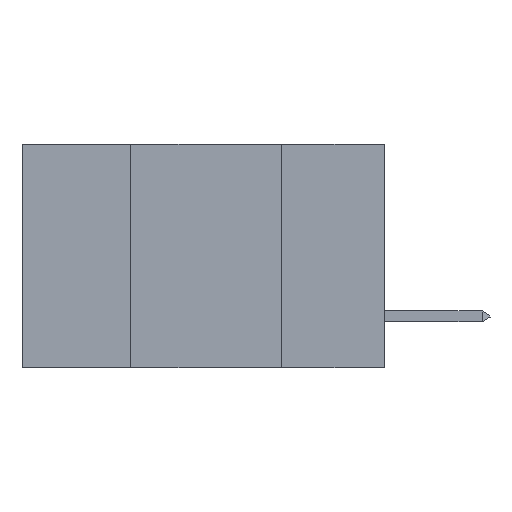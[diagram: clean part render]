
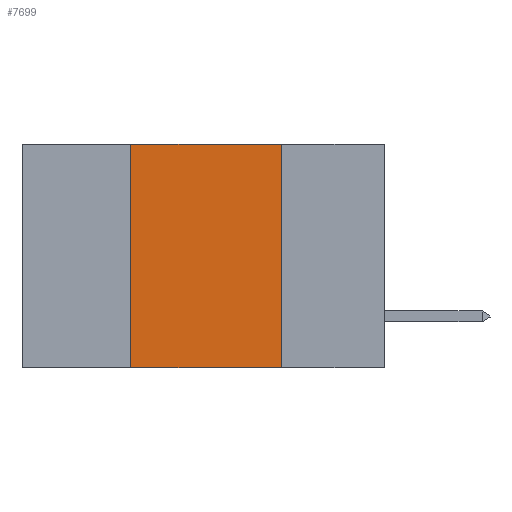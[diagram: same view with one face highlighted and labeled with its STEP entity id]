
A CAD part, left-side view. The second image highlights one B-rep face of the part: STEP entity #7699.
In plain terms, the highlighted planar face has unit normal (-1, 0, 0).
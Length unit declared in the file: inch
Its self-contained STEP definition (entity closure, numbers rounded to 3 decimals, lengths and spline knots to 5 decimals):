
#164 = DIRECTION ( 'NONE',  ( 0., -1., 0. ) ) ;
#197 = LINE ( 'NONE', #2071, #16252 ) ;
#1173 = ORIENTED_EDGE ( 'NONE', *, *, #15285, .T. ) ;
#2071 = CARTESIAN_POINT ( 'NONE',  ( 0., 0.42, 0. ) ) ;
#2928 = EDGE_CURVE ( 'NONE', #18189, #19625, #12717, .T. ) ;
#3046 = DIRECTION ( 'NONE',  ( 0., -1., 0. ) ) ;
#3427 = ORIENTED_EDGE ( 'NONE', *, *, #17826, .F. ) ;
#3479 = VECTOR ( 'NONE', #3046, 39.37008 ) ;
#3629 = DIRECTION ( 'NONE',  ( 0., 0., 1. ) ) ;
#4504 = VERTEX_POINT ( 'NONE', #11146 ) ;
#5910 = CARTESIAN_POINT ( 'NONE',  ( 0., 0.17, 0. ) ) ;
#6726 = ORIENTED_EDGE ( 'NONE', *, *, #8571, .F. ) ;
#6956 = LINE ( 'NONE', #5910, #10581 ) ;
#7299 = PLANE ( 'NONE',  #16310 ) ;
#7699 = ADVANCED_FACE ( 'NONE', ( #18673 ), #7299, .F. ) ;
#7939 = CARTESIAN_POINT ( 'NONE',  ( 0., 0.6, 0. ) ) ;
#8571 = EDGE_CURVE ( 'NONE', #4504, #18189, #197, .T. ) ;
#8852 = DIRECTION ( 'NONE',  ( 1., 0., 0. ) ) ;
#9741 = EDGE_LOOP ( 'NONE', ( #3427, #17512, #6726, #1173 ) ) ;
#9778 = VECTOR ( 'NONE', #164, 39.37008 ) ;
#10581 = VECTOR ( 'NONE', #18293, 39.37008 ) ;
#11146 = CARTESIAN_POINT ( 'NONE',  ( 0., 0.42, -0.37 ) ) ;
#12717 = LINE ( 'NONE', #7939, #3479 ) ;
#12916 = CARTESIAN_POINT ( 'NONE',  ( 0., 0.17, -0.37 ) ) ;
#13672 = VERTEX_POINT ( 'NONE', #12916 ) ;
#13927 = LINE ( 'NONE', #15679, #9778 ) ;
#15042 = DIRECTION ( 'NONE',  ( 0., 0., -1. ) ) ;
#15285 = EDGE_CURVE ( 'NONE', #4504, #13672, #13927, .T. ) ;
#15679 = CARTESIAN_POINT ( 'NONE',  ( 0., 0.6, -0.37 ) ) ;
#16252 = VECTOR ( 'NONE', #3629, 39.37008 ) ;
#16310 = AXIS2_PLACEMENT_3D ( 'NONE', #18144, #8852, #15042 ) ;
#17512 = ORIENTED_EDGE ( 'NONE', *, *, #2928, .F. ) ;
#17559 = CARTESIAN_POINT ( 'NONE',  ( 0., 0.42, 0. ) ) ;
#17826 = EDGE_CURVE ( 'NONE', #19625, #13672, #6956, .T. ) ;
#18144 = CARTESIAN_POINT ( 'NONE',  ( 0., 0.6, 0. ) ) ;
#18189 = VERTEX_POINT ( 'NONE', #17559 ) ;
#18293 = DIRECTION ( 'NONE',  ( 0., 0., -1. ) ) ;
#18576 = CARTESIAN_POINT ( 'NONE',  ( 0., 0.17, 0. ) ) ;
#18673 = FACE_OUTER_BOUND ( 'NONE', #9741, .T. ) ;
#19625 = VERTEX_POINT ( 'NONE', #18576 ) ;
